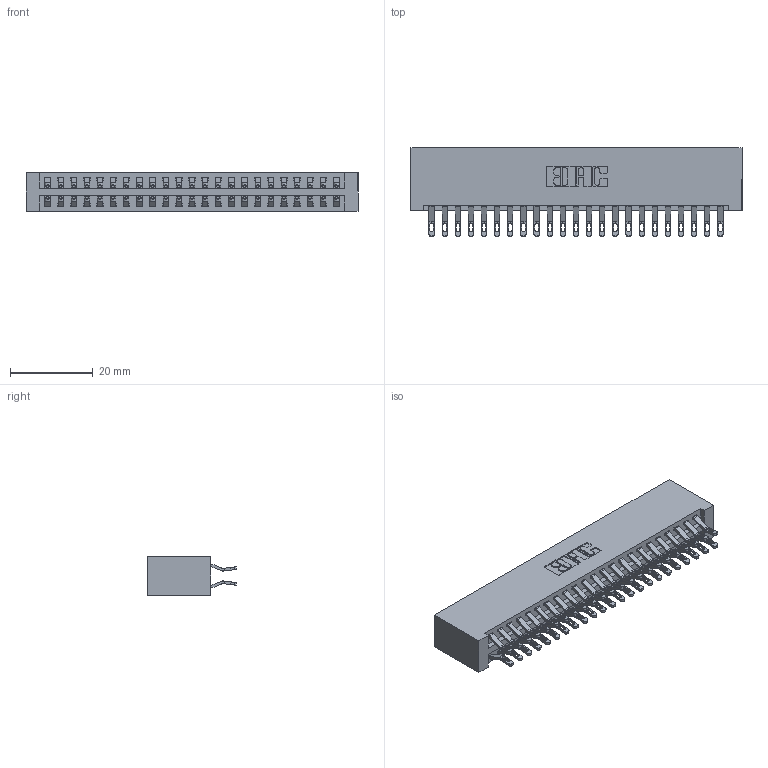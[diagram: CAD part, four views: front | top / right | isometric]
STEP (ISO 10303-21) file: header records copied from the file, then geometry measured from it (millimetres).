
FILE_DESCRIPTION (( 'STEP AP203' ), '1' );
FILE_NAME ('346-046-555-201.STEP', '2018-08-25T06:10:33', ( '' ), ( '' ), 'SwSTEP 2.0', 'SolidWorks 2016', '' );
FILE_SCHEMA (( 'CONFIG_CONTROL_DESIGN' ));
Length unit declared in the file: inch
Products named in the file (3): 346 Part_No Mounting Lugs; 345-292-001_555 Tail; 346-046-555-201
Assembly tree (47 placements, depth 2):
  346-046-555-201
    346 Part_No Mounting Lugs
    345-292-001_555 Tail  x46
Bounding box: 80.26 x 21.46 x 9.4 mm (x, y, z)
Volume: 8385.9 mm3; surface area: 11867.1 mm2
Topology: 47 solids, 47 shells, 2782 faces, 8723 edges, 5814 vertices
Faces by surface type: plane 1590, cylinder 1192
Entity records: 17617 total; most frequent: CARTESIAN_POINT 2962, ORIENTED_EDGE 2866, DIRECTION 2625, EDGE_CURVE 1433, LINE 1197, VECTOR 1197, VERTEX_POINT 954, AXIS2_PLACEMENT_3D 714
